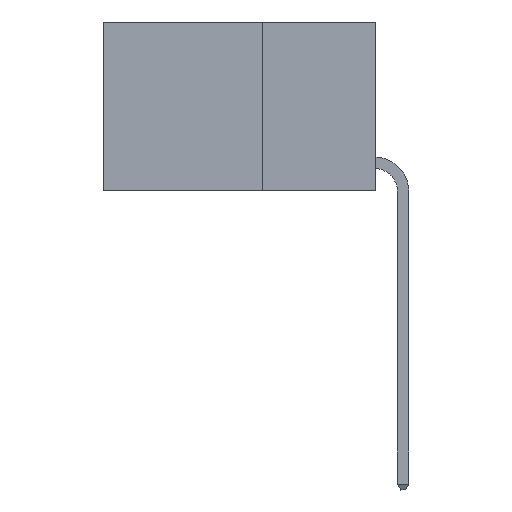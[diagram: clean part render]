
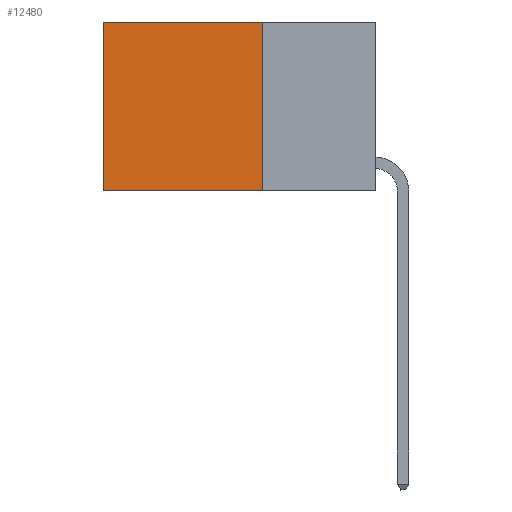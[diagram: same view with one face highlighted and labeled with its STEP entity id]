
A CAD part, left-side view. The second image highlights one B-rep face of the part: STEP entity #12480.
In plain terms, the highlighted planar face has unit normal (-1, 0, 0).
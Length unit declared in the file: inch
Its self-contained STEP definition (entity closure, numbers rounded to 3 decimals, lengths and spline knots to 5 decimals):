
#48 = EDGE_CURVE ( 'NONE', #8778, #17291, #1299, .T. ) ;
#604 = VERTEX_POINT ( 'NONE', #1847 ) ;
#1299 = LINE ( 'NONE', #7236, #3687 ) ;
#1317 = EDGE_LOOP ( 'NONE', ( #7607, #11400, #9735, #18324 ) ) ;
#1341 = CARTESIAN_POINT ( 'NONE',  ( 0.2625, 0.25, 0. ) ) ;
#1697 = VECTOR ( 'NONE', #4215, 39.37008 ) ;
#1705 = EDGE_CURVE ( 'NONE', #604, #9204, #18987, .T. ) ;
#1847 = CARTESIAN_POINT ( 'NONE',  ( 0.2625, 0.25, -0.37 ) ) ;
#3683 = FACE_OUTER_BOUND ( 'NONE', #1317, .T. ) ;
#3687 = VECTOR ( 'NONE', #14818, 39.37008 ) ;
#4215 = DIRECTION ( 'NONE',  ( 0., 0., -1. ) ) ;
#4332 = CARTESIAN_POINT ( 'NONE',  ( 0.2625, 0.25, 0. ) ) ;
#5268 = DIRECTION ( 'NONE',  ( 0., 1., 0. ) ) ;
#5307 = PLANE ( 'NONE',  #13568 ) ;
#7236 = CARTESIAN_POINT ( 'NONE',  ( 0.2625, 0.25, 0. ) ) ;
#7469 = CARTESIAN_POINT ( 'NONE',  ( 0.2625, 0.6, 0. ) ) ;
#7607 = ORIENTED_EDGE ( 'NONE', *, *, #19376, .T. ) ;
#8778 = VERTEX_POINT ( 'NONE', #4332 ) ;
#9204 = VERTEX_POINT ( 'NONE', #10294 ) ;
#9735 = ORIENTED_EDGE ( 'NONE', *, *, #10676, .F. ) ;
#10294 = CARTESIAN_POINT ( 'NONE',  ( 0.2625, 0.6, -0.37 ) ) ;
#10676 = EDGE_CURVE ( 'NONE', #8778, #604, #17083, .T. ) ;
#11400 = ORIENTED_EDGE ( 'NONE', *, *, #1705, .F. ) ;
#11604 = CARTESIAN_POINT ( 'NONE',  ( 0.2625, 0.25, 0. ) ) ;
#12142 = LINE ( 'NONE', #7469, #1697 ) ;
#12480 = ADVANCED_FACE ( 'NONE', ( #3683 ), #5307, .F. ) ;
#13027 = VECTOR ( 'NONE', #5268, 39.37008 ) ;
#13098 = CARTESIAN_POINT ( 'NONE',  ( 0.2625, 0.25, -0.37 ) ) ;
#13568 = AXIS2_PLACEMENT_3D ( 'NONE', #11604, #19219, #16249 ) ;
#13839 = VECTOR ( 'NONE', #14058, 39.37008 ) ;
#14058 = DIRECTION ( 'NONE',  ( 0., 0., -1. ) ) ;
#14818 = DIRECTION ( 'NONE',  ( 0., 1., 0. ) ) ;
#15607 = CARTESIAN_POINT ( 'NONE',  ( 0.2625, 0.6, 0. ) ) ;
#16249 = DIRECTION ( 'NONE',  ( 0., 0., -1. ) ) ;
#17083 = LINE ( 'NONE', #1341, #13839 ) ;
#17291 = VERTEX_POINT ( 'NONE', #15607 ) ;
#18324 = ORIENTED_EDGE ( 'NONE', *, *, #48, .T. ) ;
#18987 = LINE ( 'NONE', #13098, #13027 ) ;
#19219 = DIRECTION ( 'NONE',  ( 1., 0., 0. ) ) ;
#19376 = EDGE_CURVE ( 'NONE', #17291, #9204, #12142, .T. ) ;
